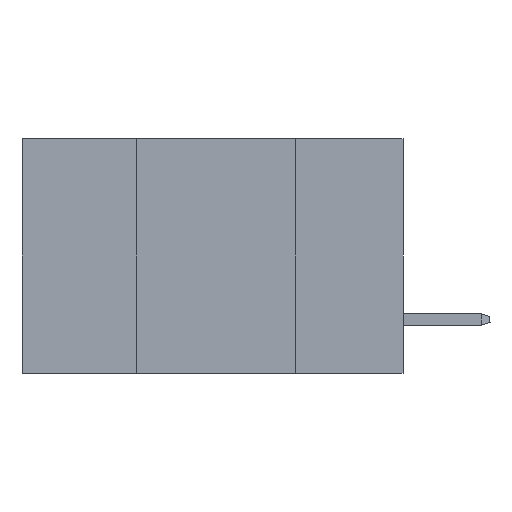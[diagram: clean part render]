
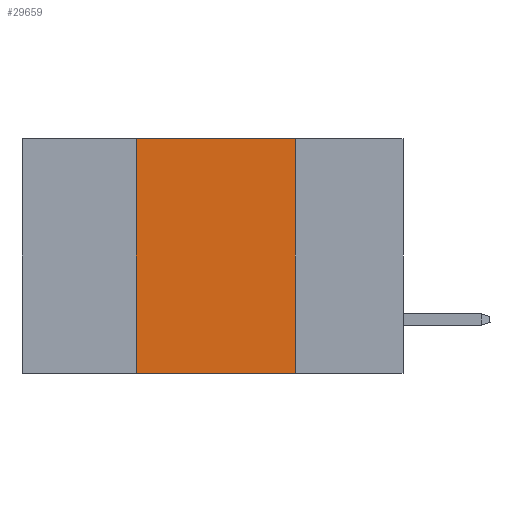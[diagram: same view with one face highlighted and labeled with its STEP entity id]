
A CAD part, left-side view. The second image highlights one B-rep face of the part: STEP entity #29659.
In plain terms, the highlighted planar face has unit normal (-1, 0, 0).
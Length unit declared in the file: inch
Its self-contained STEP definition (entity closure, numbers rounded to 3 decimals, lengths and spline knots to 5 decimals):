
#3015 = CARTESIAN_POINT ( 'NONE',  ( 0., 0.6, 0. ) ) ;
#3430 = EDGE_CURVE ( 'NONE', #17376, #23830, #17480, .T. ) ;
#4992 = ORIENTED_EDGE ( 'NONE', *, *, #3430, .F. ) ;
#5005 = VECTOR ( 'NONE', #23749, 39.37008 ) ;
#5370 = ORIENTED_EDGE ( 'NONE', *, *, #24681, .F. ) ;
#6742 = CARTESIAN_POINT ( 'NONE',  ( 0., 0.17, -0.37 ) ) ;
#6923 = CARTESIAN_POINT ( 'NONE',  ( 0., 0.6, 0. ) ) ;
#8414 = DIRECTION ( 'NONE',  ( 0., -1., 0. ) ) ;
#9755 = CARTESIAN_POINT ( 'NONE',  ( 0., 0.42, -0.37 ) ) ;
#11343 = CARTESIAN_POINT ( 'NONE',  ( 0., 0.17, 0. ) ) ;
#11499 = DIRECTION ( 'NONE',  ( 1., 0., 0. ) ) ;
#12006 = CARTESIAN_POINT ( 'NONE',  ( 0., 0.42, 0. ) ) ;
#12747 = VECTOR ( 'NONE', #17500, 39.37008 ) ;
#13737 = EDGE_LOOP ( 'NONE', ( #5370, #4992, #17945, #24635 ) ) ;
#14987 = EDGE_CURVE ( 'NONE', #29316, #22704, #32517, .T. ) ;
#16262 = VECTOR ( 'NONE', #8414, 39.37008 ) ;
#16770 = PLANE ( 'NONE',  #27697 ) ;
#17376 = VERTEX_POINT ( 'NONE', #12006 ) ;
#17480 = LINE ( 'NONE', #6923, #31513 ) ;
#17500 = DIRECTION ( 'NONE',  ( 0., 0., 1. ) ) ;
#17945 = ORIENTED_EDGE ( 'NONE', *, *, #22261, .F. ) ;
#19038 = DIRECTION ( 'NONE',  ( 0., 0., -1. ) ) ;
#20121 = LINE ( 'NONE', #30890, #12747 ) ;
#20796 = DIRECTION ( 'NONE',  ( 0., -1., 0. ) ) ;
#21501 = FACE_OUTER_BOUND ( 'NONE', #13737, .T. ) ;
#22261 = EDGE_CURVE ( 'NONE', #29316, #17376, #20121, .T. ) ;
#22704 = VERTEX_POINT ( 'NONE', #6742 ) ;
#22870 = LINE ( 'NONE', #33636, #5005 ) ;
#23749 = DIRECTION ( 'NONE',  ( 0., 0., -1. ) ) ;
#23830 = VERTEX_POINT ( 'NONE', #11343 ) ;
#24635 = ORIENTED_EDGE ( 'NONE', *, *, #14987, .T. ) ;
#24681 = EDGE_CURVE ( 'NONE', #23830, #22704, #22870, .T. ) ;
#27697 = AXIS2_PLACEMENT_3D ( 'NONE', #3015, #11499, #19038 ) ;
#29316 = VERTEX_POINT ( 'NONE', #9755 ) ;
#29659 = ADVANCED_FACE ( 'NONE', ( #21501 ), #16770, .F. ) ;
#30033 = CARTESIAN_POINT ( 'NONE',  ( 0., 0.6, -0.37 ) ) ;
#30890 = CARTESIAN_POINT ( 'NONE',  ( 0., 0.42, 0. ) ) ;
#31513 = VECTOR ( 'NONE', #20796, 39.37008 ) ;
#32517 = LINE ( 'NONE', #30033, #16262 ) ;
#33636 = CARTESIAN_POINT ( 'NONE',  ( 0., 0.17, 0. ) ) ;
